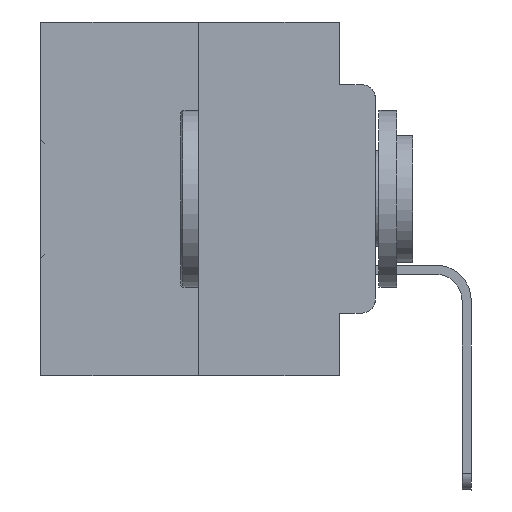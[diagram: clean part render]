
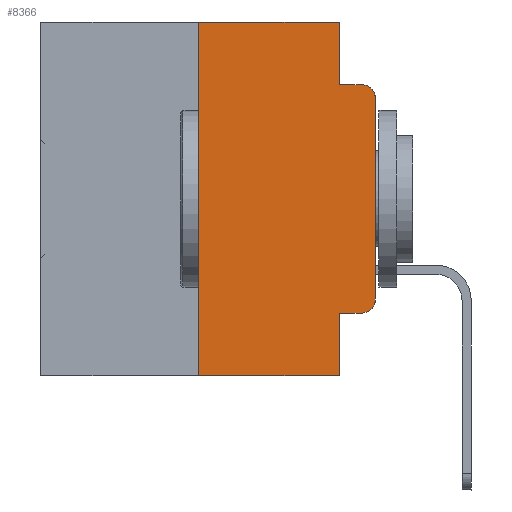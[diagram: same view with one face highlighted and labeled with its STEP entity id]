
A CAD part, left-side view. The second image highlights one B-rep face of the part: STEP entity #8366.
In plain terms, the highlighted planar face has unit normal (-1, 0, 0).
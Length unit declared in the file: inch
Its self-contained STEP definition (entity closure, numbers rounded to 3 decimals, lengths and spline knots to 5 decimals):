
#278 = DIRECTION ( 'NONE',  ( 0., 0., -1. ) ) ;
#678 = VERTEX_POINT ( 'NONE', #6010 ) ;
#730 = EDGE_CURVE ( 'NONE', #11149, #678, #7836, .T. ) ;
#951 = CARTESIAN_POINT ( 'NONE',  ( 0., 0.25, 0. ) ) ;
#1190 = VECTOR ( 'NONE', #17617, 39.37008 ) ;
#1612 = ORIENTED_EDGE ( 'NONE', *, *, #17588, .F. ) ;
#1976 = CARTESIAN_POINT ( 'NONE',  ( 0., 0.02, -0.0885 ) ) ;
#2380 = VERTEX_POINT ( 'NONE', #6271 ) ;
#2780 = ORIENTED_EDGE ( 'NONE', *, *, #20652, .T. ) ;
#2848 = CARTESIAN_POINT ( 'NONE',  ( 0., 0.051, -0.0885 ) ) ;
#2919 = VECTOR ( 'NONE', #19703, 39.37008 ) ;
#3439 = DIRECTION ( 'NONE',  ( -1., 0., 0. ) ) ;
#3791 = CARTESIAN_POINT ( 'NONE',  ( 0., 0., -0.3915 ) ) ;
#5033 = EDGE_CURVE ( 'NONE', #2380, #15990, #27979, .T. ) ;
#5264 = CARTESIAN_POINT ( 'NONE',  ( 0., 0.473, -0.5 ) ) ;
#5696 = DIRECTION ( 'NONE',  ( -1., 0., 0. ) ) ;
#5720 = VECTOR ( 'NONE', #31138, 39.37008 ) ;
#5942 = EDGE_CURVE ( 'NONE', #11149, #24972, #14156, .T. ) ;
#6010 = CARTESIAN_POINT ( 'NONE',  ( 0., 0.02, -0.4115 ) ) ;
#6176 = VECTOR ( 'NONE', #23601, 39.37008 ) ;
#6271 = CARTESIAN_POINT ( 'NONE',  ( 0., 0.051, 0. ) ) ;
#6320 = CARTESIAN_POINT ( 'NONE',  ( 0., 0.051, -0.4115 ) ) ;
#6706 = CIRCLE ( 'NONE', #25809, 0.02 ) ;
#6773 = DIRECTION ( 'NONE',  ( 0., -1., 0. ) ) ;
#6970 = VECTOR ( 'NONE', #6773, 39.37008 ) ;
#7836 = LINE ( 'NONE', #17064, #6970 ) ;
#8007 = EDGE_LOOP ( 'NONE', ( #32240, #26002, #33098, #17541, #1612, #22801, #12900, #28671, #15363, #2780 ) ) ;
#8366 = ADVANCED_FACE ( 'NONE', ( #28959 ), #10479, .F. ) ;
#8476 = AXIS2_PLACEMENT_3D ( 'NONE', #11359, #3439, #27077 ) ;
#8596 = LINE ( 'NONE', #5264, #32841 ) ;
#8748 = LINE ( 'NONE', #14516, #28190 ) ;
#9798 = CIRCLE ( 'NONE', #8476, 0.02 ) ;
#10479 = PLANE ( 'NONE',  #28563 ) ;
#10590 = DIRECTION ( 'NONE',  ( 1., 0., 0. ) ) ;
#11149 = VERTEX_POINT ( 'NONE', #6320 ) ;
#11359 = CARTESIAN_POINT ( 'NONE',  ( 0., 0.02, -0.1085 ) ) ;
#11777 = CARTESIAN_POINT ( 'NONE',  ( 0., 0.051, -0.0885 ) ) ;
#12531 = CARTESIAN_POINT ( 'NONE',  ( 0., 0.051, -0.5 ) ) ;
#12668 = EDGE_CURVE ( 'NONE', #19382, #18917, #8748, .T. ) ;
#12900 = ORIENTED_EDGE ( 'NONE', *, *, #31956, .T. ) ;
#13574 = VERTEX_POINT ( 'NONE', #31097 ) ;
#14156 = LINE ( 'NONE', #30738, #1190 ) ;
#14516 = CARTESIAN_POINT ( 'NONE',  ( 0., 0., 0. ) ) ;
#14915 = CARTESIAN_POINT ( 'NONE',  ( 0., 0., -0.1085 ) ) ;
#15363 = ORIENTED_EDGE ( 'NONE', *, *, #730, .T. ) ;
#15980 = CARTESIAN_POINT ( 'NONE',  ( 0., 0.051, 0. ) ) ;
#15990 = VERTEX_POINT ( 'NONE', #2848 ) ;
#16098 = DIRECTION ( 'NONE',  ( 0., 0., -1. ) ) ;
#16342 = LINE ( 'NONE', #32730, #31348 ) ;
#17064 = CARTESIAN_POINT ( 'NONE',  ( 0., 0.051, -0.4115 ) ) ;
#17541 = ORIENTED_EDGE ( 'NONE', *, *, #5033, .F. ) ;
#17588 = EDGE_CURVE ( 'NONE', #23963, #2380, #16342, .T. ) ;
#17617 = DIRECTION ( 'NONE',  ( 0., 0., -1. ) ) ;
#18491 = CARTESIAN_POINT ( 'NONE',  ( 0., 0.25, 0. ) ) ;
#18917 = VERTEX_POINT ( 'NONE', #14915 ) ;
#19095 = LINE ( 'NONE', #11777, #2919 ) ;
#19115 = LINE ( 'NONE', #18491, #6176 ) ;
#19382 = VERTEX_POINT ( 'NONE', #3791 ) ;
#19499 = VERTEX_POINT ( 'NONE', #1976 ) ;
#19703 = DIRECTION ( 'NONE',  ( 0., -1., 0. ) ) ;
#19716 = DIRECTION ( 'NONE',  ( 0., 0., 1. ) ) ;
#20652 = EDGE_CURVE ( 'NONE', #678, #19382, #6706, .T. ) ;
#21280 = CARTESIAN_POINT ( 'NONE',  ( 0., 0.02, -0.3915 ) ) ;
#22801 = ORIENTED_EDGE ( 'NONE', *, *, #33405, .F. ) ;
#23601 = DIRECTION ( 'NONE',  ( 0., 0., 1. ) ) ;
#23963 = VERTEX_POINT ( 'NONE', #951 ) ;
#24972 = VERTEX_POINT ( 'NONE', #12531 ) ;
#25809 = AXIS2_PLACEMENT_3D ( 'NONE', #21280, #5696, #16098 ) ;
#26002 = ORIENTED_EDGE ( 'NONE', *, *, #32277, .T. ) ;
#26110 = CARTESIAN_POINT ( 'NONE',  ( 0., 0.473, 0. ) ) ;
#27077 = DIRECTION ( 'NONE',  ( 0., 0., -1. ) ) ;
#27667 = DIRECTION ( 'NONE',  ( 0., -1., 0. ) ) ;
#27979 = LINE ( 'NONE', #15980, #5720 ) ;
#28190 = VECTOR ( 'NONE', #19716, 39.37008 ) ;
#28563 = AXIS2_PLACEMENT_3D ( 'NONE', #26110, #10590, #278 ) ;
#28671 = ORIENTED_EDGE ( 'NONE', *, *, #5942, .F. ) ;
#28959 = FACE_OUTER_BOUND ( 'NONE', #8007, .T. ) ;
#30738 = CARTESIAN_POINT ( 'NONE',  ( 0., 0.051, 0. ) ) ;
#30942 = DIRECTION ( 'NONE',  ( 0., -1., 0. ) ) ;
#31097 = CARTESIAN_POINT ( 'NONE',  ( 0., 0.25, -0.5 ) ) ;
#31138 = DIRECTION ( 'NONE',  ( 0., 0., -1. ) ) ;
#31348 = VECTOR ( 'NONE', #27667, 39.37008 ) ;
#31956 = EDGE_CURVE ( 'NONE', #13574, #24972, #8596, .T. ) ;
#32240 = ORIENTED_EDGE ( 'NONE', *, *, #12668, .T. ) ;
#32277 = EDGE_CURVE ( 'NONE', #18917, #19499, #9798, .T. ) ;
#32301 = EDGE_CURVE ( 'NONE', #15990, #19499, #19095, .T. ) ;
#32730 = CARTESIAN_POINT ( 'NONE',  ( 0., 0.473, 0. ) ) ;
#32841 = VECTOR ( 'NONE', #30942, 39.37008 ) ;
#33098 = ORIENTED_EDGE ( 'NONE', *, *, #32301, .F. ) ;
#33405 = EDGE_CURVE ( 'NONE', #13574, #23963, #19115, .T. ) ;
